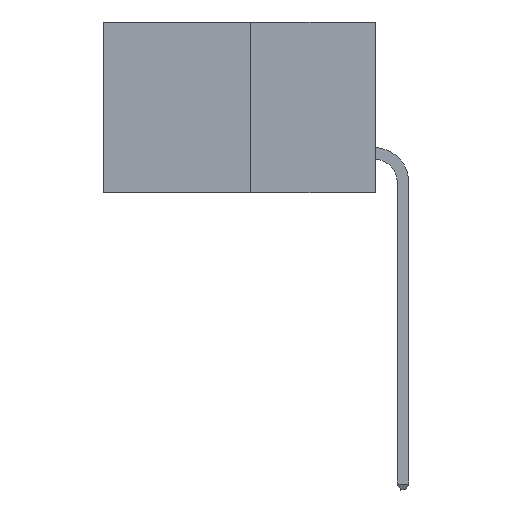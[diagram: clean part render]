
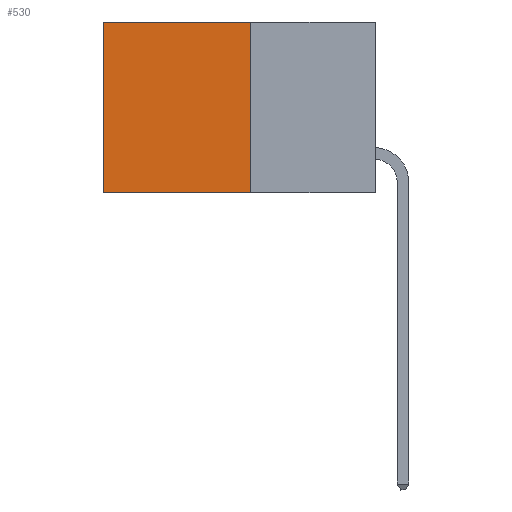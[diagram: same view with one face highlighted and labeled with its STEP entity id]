
A CAD part, left-side view. The second image highlights one B-rep face of the part: STEP entity #530.
In plain terms, the highlighted planar face has unit normal (-1, 0, 0).
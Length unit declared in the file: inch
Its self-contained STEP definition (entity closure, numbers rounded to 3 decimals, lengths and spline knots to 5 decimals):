
#214 = CARTESIAN_POINT ( 'NONE',  ( 0.277, 0.59, -0.37 ) ) ;
#484 = ORIENTED_EDGE ( 'NONE', *, *, #9727, .T. ) ;
#530 = ADVANCED_FACE ( 'NONE', ( #14951 ), #11928, .F. ) ;
#555 = CARTESIAN_POINT ( 'NONE',  ( 0.277, 0.59, -0.37 ) ) ;
#1208 = DIRECTION ( 'NONE',  ( 0., 1., 0. ) ) ;
#1677 = EDGE_LOOP ( 'NONE', ( #484, #14681, #11089, #2837 ) ) ;
#2484 = LINE ( 'NONE', #6300, #14339 ) ;
#2837 = ORIENTED_EDGE ( 'NONE', *, *, #12017, .T. ) ;
#3294 = CARTESIAN_POINT ( 'NONE',  ( 0.277, 0.27, 0. ) ) ;
#3982 = EDGE_CURVE ( 'NONE', #13161, #9913, #10222, .T. ) ;
#5155 = CARTESIAN_POINT ( 'NONE',  ( 0.277, 0.27, -0.37 ) ) ;
#5490 = CARTESIAN_POINT ( 'NONE',  ( 0.277, 0.27, 0. ) ) ;
#6300 = CARTESIAN_POINT ( 'NONE',  ( 0.277, 0.27, -0.37 ) ) ;
#6571 = DIRECTION ( 'NONE',  ( 0., 0., -1. ) ) ;
#7079 = DIRECTION ( 'NONE',  ( 0., 0., -1. ) ) ;
#8146 = EDGE_CURVE ( 'NONE', #9913, #12655, #2484, .T. ) ;
#8435 = VERTEX_POINT ( 'NONE', #11453 ) ;
#9364 = AXIS2_PLACEMENT_3D ( 'NONE', #10243, #9536, #14578 ) ;
#9536 = DIRECTION ( 'NONE',  ( 1., 0., 0. ) ) ;
#9727 = EDGE_CURVE ( 'NONE', #8435, #12655, #13279, .T. ) ;
#9913 = VERTEX_POINT ( 'NONE', #13826 ) ;
#10222 = LINE ( 'NONE', #5155, #12535 ) ;
#10243 = CARTESIAN_POINT ( 'NONE',  ( 0.277, 0.27, -0.37 ) ) ;
#10871 = VECTOR ( 'NONE', #13898, 39.37008 ) ;
#11089 = ORIENTED_EDGE ( 'NONE', *, *, #3982, .F. ) ;
#11453 = CARTESIAN_POINT ( 'NONE',  ( 0.277, 0.59, 0. ) ) ;
#11928 = PLANE ( 'NONE',  #9364 ) ;
#12017 = EDGE_CURVE ( 'NONE', #13161, #8435, #13863, .T. ) ;
#12535 = VECTOR ( 'NONE', #7079, 39.37008 ) ;
#12655 = VERTEX_POINT ( 'NONE', #555 ) ;
#13161 = VERTEX_POINT ( 'NONE', #5490 ) ;
#13279 = LINE ( 'NONE', #214, #14121 ) ;
#13826 = CARTESIAN_POINT ( 'NONE',  ( 0.277, 0.27, -0.37 ) ) ;
#13863 = LINE ( 'NONE', #3294, #10871 ) ;
#13898 = DIRECTION ( 'NONE',  ( 0., 1., 0. ) ) ;
#14121 = VECTOR ( 'NONE', #6571, 39.37008 ) ;
#14339 = VECTOR ( 'NONE', #1208, 39.37008 ) ;
#14578 = DIRECTION ( 'NONE',  ( 0., 0., -1. ) ) ;
#14681 = ORIENTED_EDGE ( 'NONE', *, *, #8146, .F. ) ;
#14951 = FACE_OUTER_BOUND ( 'NONE', #1677, .T. ) ;
